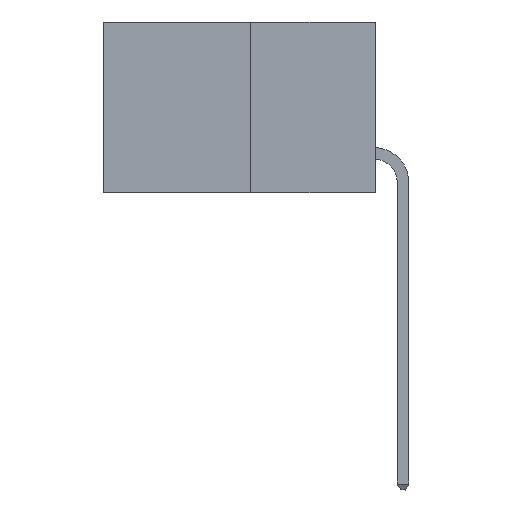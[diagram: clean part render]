
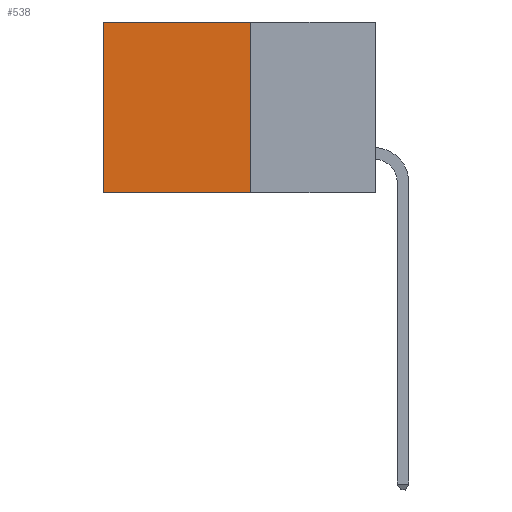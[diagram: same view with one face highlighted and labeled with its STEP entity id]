
A CAD part, left-side view. The second image highlights one B-rep face of the part: STEP entity #538.
In plain terms, the highlighted planar face has unit normal (-1, 0, 0).
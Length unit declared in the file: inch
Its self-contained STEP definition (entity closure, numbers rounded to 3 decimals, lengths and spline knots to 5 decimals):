
#538 = ADVANCED_FACE ( 'NONE', ( #10311 ), #8204, .F. ) ;
#579 = VECTOR ( 'NONE', #1812, 39.37008 ) ;
#1457 = EDGE_LOOP ( 'NONE', ( #7468, #12157, #7496, #6116 ) ) ;
#1664 = CARTESIAN_POINT ( 'NONE',  ( 0.277, 0.27, -0.37 ) ) ;
#1812 = DIRECTION ( 'NONE',  ( 0., 1., 0. ) ) ;
#2018 = VERTEX_POINT ( 'NONE', #5528 ) ;
#2647 = EDGE_CURVE ( 'NONE', #8254, #2018, #8044, .T. ) ;
#3027 = CARTESIAN_POINT ( 'NONE',  ( 0.277, 0.27, -0.37 ) ) ;
#3050 = LINE ( 'NONE', #15719, #5754 ) ;
#3091 = CARTESIAN_POINT ( 'NONE',  ( 0.277, 0.59, -0.37 ) ) ;
#3202 = CARTESIAN_POINT ( 'NONE',  ( 0.277, 0.27, 0. ) ) ;
#3638 = EDGE_CURVE ( 'NONE', #8254, #16442, #3050, .T. ) ;
#3648 = CARTESIAN_POINT ( 'NONE',  ( 0.277, 0.59, -0.37 ) ) ;
#4556 = VECTOR ( 'NONE', #10344, 39.37008 ) ;
#5239 = VERTEX_POINT ( 'NONE', #3091 ) ;
#5421 = EDGE_CURVE ( 'NONE', #2018, #5239, #13119, .T. ) ;
#5528 = CARTESIAN_POINT ( 'NONE',  ( 0.277, 0.27, -0.37 ) ) ;
#5754 = VECTOR ( 'NONE', #15772, 39.37008 ) ;
#6116 = ORIENTED_EDGE ( 'NONE', *, *, #3638, .T. ) ;
#7468 = ORIENTED_EDGE ( 'NONE', *, *, #11948, .T. ) ;
#7496 = ORIENTED_EDGE ( 'NONE', *, *, #2647, .F. ) ;
#8044 = LINE ( 'NONE', #3027, #4556 ) ;
#8204 = PLANE ( 'NONE',  #13405 ) ;
#8254 = VERTEX_POINT ( 'NONE', #3202 ) ;
#8791 = CARTESIAN_POINT ( 'NONE',  ( 0.277, 0.27, -0.37 ) ) ;
#9219 = DIRECTION ( 'NONE',  ( 1., 0., 0. ) ) ;
#10180 = CARTESIAN_POINT ( 'NONE',  ( 0.277, 0.59, 0. ) ) ;
#10311 = FACE_OUTER_BOUND ( 'NONE', #1457, .T. ) ;
#10344 = DIRECTION ( 'NONE',  ( 0., 0., -1. ) ) ;
#11309 = DIRECTION ( 'NONE',  ( 0., 0., -1. ) ) ;
#11948 = EDGE_CURVE ( 'NONE', #16442, #5239, #13812, .T. ) ;
#12157 = ORIENTED_EDGE ( 'NONE', *, *, #5421, .F. ) ;
#12417 = DIRECTION ( 'NONE',  ( 0., 0., -1. ) ) ;
#13037 = VECTOR ( 'NONE', #11309, 39.37008 ) ;
#13119 = LINE ( 'NONE', #1664, #579 ) ;
#13405 = AXIS2_PLACEMENT_3D ( 'NONE', #8791, #9219, #12417 ) ;
#13812 = LINE ( 'NONE', #3648, #13037 ) ;
#15719 = CARTESIAN_POINT ( 'NONE',  ( 0.277, 0.27, 0. ) ) ;
#15772 = DIRECTION ( 'NONE',  ( 0., 1., 0. ) ) ;
#16442 = VERTEX_POINT ( 'NONE', #10180 ) ;
